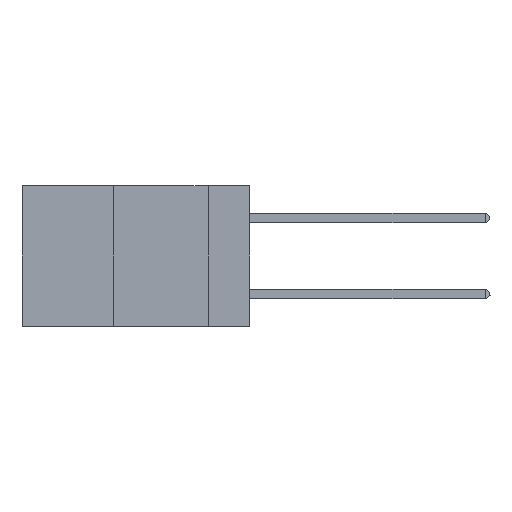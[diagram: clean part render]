
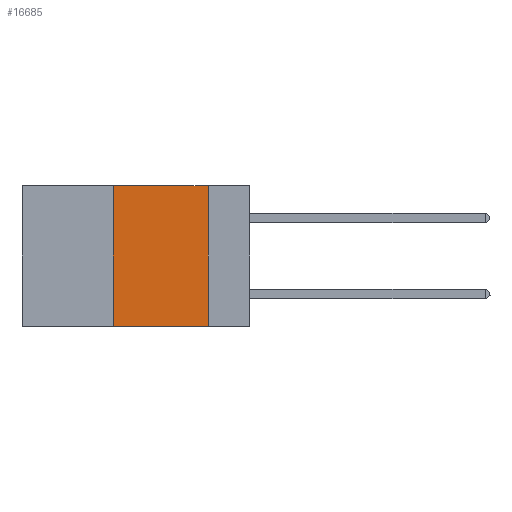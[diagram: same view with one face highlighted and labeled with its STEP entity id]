
A CAD part, left-side view. The second image highlights one B-rep face of the part: STEP entity #16685.
In plain terms, the highlighted planar face has unit normal (-1, 0, 0).
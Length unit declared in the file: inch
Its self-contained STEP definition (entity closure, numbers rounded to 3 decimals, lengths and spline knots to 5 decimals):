
#200 = ORIENTED_EDGE ( 'NONE', *, *, #10213, .F. ) ;
#511 = VECTOR ( 'NONE', #8162, 39.37008 ) ;
#2200 = CARTESIAN_POINT ( 'NONE',  ( 0., 0.36, 0. ) ) ;
#4550 = VECTOR ( 'NONE', #31954, 39.37008 ) ;
#6019 = DIRECTION ( 'NONE',  ( 1., 0., 0. ) ) ;
#6268 = CARTESIAN_POINT ( 'NONE',  ( 0., 0.11, 0. ) ) ;
#6274 = PLANE ( 'NONE',  #27233 ) ;
#8068 = VERTEX_POINT ( 'NONE', #30042 ) ;
#8162 = DIRECTION ( 'NONE',  ( 0., 0., 1. ) ) ;
#9043 = CARTESIAN_POINT ( 'NONE',  ( 0., 0.36, -0.37 ) ) ;
#10213 = EDGE_CURVE ( 'NONE', #35956, #21075, #29665, .T. ) ;
#12491 = ORIENTED_EDGE ( 'NONE', *, *, #14887, .F. ) ;
#12923 = DIRECTION ( 'NONE',  ( 0., -1., 0. ) ) ;
#14887 = EDGE_CURVE ( 'NONE', #16875, #8068, #30322, .T. ) ;
#16403 = CARTESIAN_POINT ( 'NONE',  ( 0., 0.11, 0. ) ) ;
#16684 = ORIENTED_EDGE ( 'NONE', *, *, #21068, .F. ) ;
#16685 = ADVANCED_FACE ( 'NONE', ( #33080 ), #6274, .F. ) ;
#16875 = VERTEX_POINT ( 'NONE', #16403 ) ;
#17523 = CARTESIAN_POINT ( 'NONE',  ( 0., 0.6, -0.37 ) ) ;
#17768 = VECTOR ( 'NONE', #39322, 39.37008 ) ;
#19142 = CARTESIAN_POINT ( 'NONE',  ( 0., 0.36, 0. ) ) ;
#21068 = EDGE_CURVE ( 'NONE', #21075, #16875, #28999, .T. ) ;
#21075 = VERTEX_POINT ( 'NONE', #19142 ) ;
#21631 = VECTOR ( 'NONE', #12923, 39.37008 ) ;
#21933 = EDGE_CURVE ( 'NONE', #35956, #8068, #38249, .T. ) ;
#24315 = EDGE_LOOP ( 'NONE', ( #12491, #16684, #200, #29706 ) ) ;
#27233 = AXIS2_PLACEMENT_3D ( 'NONE', #34019, #6019, #27993 ) ;
#27993 = DIRECTION ( 'NONE',  ( 0., 0., -1. ) ) ;
#28999 = LINE ( 'NONE', #38071, #21631 ) ;
#29665 = LINE ( 'NONE', #2200, #511 ) ;
#29706 = ORIENTED_EDGE ( 'NONE', *, *, #21933, .T. ) ;
#30042 = CARTESIAN_POINT ( 'NONE',  ( 0., 0.11, -0.37 ) ) ;
#30322 = LINE ( 'NONE', #6268, #4550 ) ;
#31954 = DIRECTION ( 'NONE',  ( 0., 0., -1. ) ) ;
#33080 = FACE_OUTER_BOUND ( 'NONE', #24315, .T. ) ;
#34019 = CARTESIAN_POINT ( 'NONE',  ( 0., 0.6, 0. ) ) ;
#35956 = VERTEX_POINT ( 'NONE', #9043 ) ;
#38071 = CARTESIAN_POINT ( 'NONE',  ( 0., 0.6, 0. ) ) ;
#38249 = LINE ( 'NONE', #17523, #17768 ) ;
#39322 = DIRECTION ( 'NONE',  ( 0., -1., 0. ) ) ;
